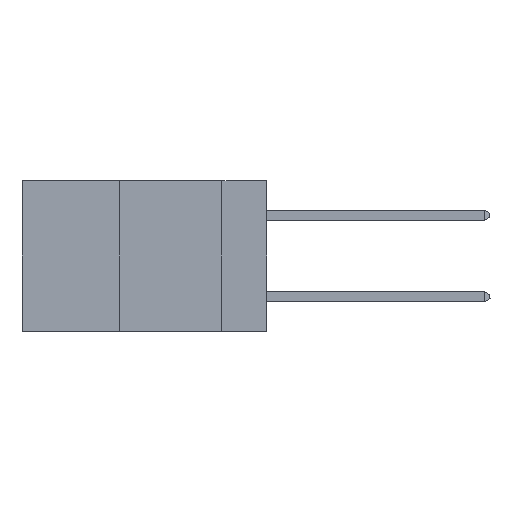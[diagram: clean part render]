
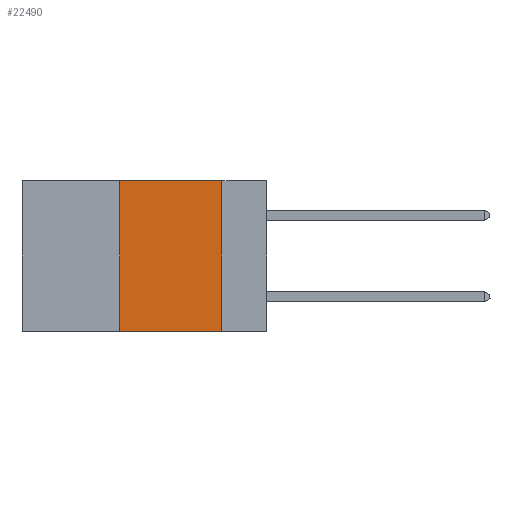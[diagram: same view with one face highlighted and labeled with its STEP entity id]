
A CAD part, left-side view. The second image highlights one B-rep face of the part: STEP entity #22490.
In plain terms, the highlighted planar face has unit normal (-1, 0, 0).
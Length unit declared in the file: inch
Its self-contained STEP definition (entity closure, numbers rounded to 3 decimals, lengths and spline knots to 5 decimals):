
#367 = VECTOR ( 'NONE', #22513, 39.37008 ) ;
#1401 = CARTESIAN_POINT ( 'NONE',  ( 0., 0.6, -0.37 ) ) ;
#1449 = CARTESIAN_POINT ( 'NONE',  ( 0., 0.11, 0. ) ) ;
#2160 = DIRECTION ( 'NONE',  ( 0., 0., -1. ) ) ;
#3634 = EDGE_CURVE ( 'NONE', #8290, #9306, #16051, .T. ) ;
#5881 = CARTESIAN_POINT ( 'NONE',  ( 0., 0.6, 0. ) ) ;
#7164 = EDGE_CURVE ( 'NONE', #9306, #13110, #24698, .T. ) ;
#7199 = FACE_OUTER_BOUND ( 'NONE', #22809, .T. ) ;
#7933 = DIRECTION ( 'NONE',  ( 1., 0., 0. ) ) ;
#8290 = VERTEX_POINT ( 'NONE', #11696 ) ;
#8476 = VECTOR ( 'NONE', #19211, 39.37008 ) ;
#8599 = CARTESIAN_POINT ( 'NONE',  ( 0., 0.11, -0.37 ) ) ;
#9306 = VERTEX_POINT ( 'NONE', #1449 ) ;
#9375 = CARTESIAN_POINT ( 'NONE',  ( 0., 0.36, -0.37 ) ) ;
#11696 = CARTESIAN_POINT ( 'NONE',  ( 0., 0.36, 0. ) ) ;
#12373 = CARTESIAN_POINT ( 'NONE',  ( 0., 0.11, 0. ) ) ;
#12525 = VECTOR ( 'NONE', #17699, 39.37008 ) ;
#13110 = VERTEX_POINT ( 'NONE', #8599 ) ;
#14006 = EDGE_CURVE ( 'NONE', #24593, #8290, #17898, .T. ) ;
#14942 = VECTOR ( 'NONE', #2160, 39.37008 ) ;
#15352 = EDGE_CURVE ( 'NONE', #24593, #13110, #22393, .T. ) ;
#16051 = LINE ( 'NONE', #23934, #367 ) ;
#17699 = DIRECTION ( 'NONE',  ( 0., -1., 0. ) ) ;
#17898 = LINE ( 'NONE', #21150, #8476 ) ;
#17974 = PLANE ( 'NONE',  #25575 ) ;
#19211 = DIRECTION ( 'NONE',  ( 0., 0., 1. ) ) ;
#20275 = ORIENTED_EDGE ( 'NONE', *, *, #3634, .F. ) ;
#20504 = ORIENTED_EDGE ( 'NONE', *, *, #7164, .F. ) ;
#21150 = CARTESIAN_POINT ( 'NONE',  ( 0., 0.36, 0. ) ) ;
#21880 = DIRECTION ( 'NONE',  ( 0., 0., -1. ) ) ;
#22393 = LINE ( 'NONE', #1401, #12525 ) ;
#22490 = ADVANCED_FACE ( 'NONE', ( #7199 ), #17974, .F. ) ;
#22513 = DIRECTION ( 'NONE',  ( 0., -1., 0. ) ) ;
#22708 = ORIENTED_EDGE ( 'NONE', *, *, #15352, .T. ) ;
#22809 = EDGE_LOOP ( 'NONE', ( #20504, #20275, #22950, #22708 ) ) ;
#22950 = ORIENTED_EDGE ( 'NONE', *, *, #14006, .F. ) ;
#23934 = CARTESIAN_POINT ( 'NONE',  ( 0., 0.6, 0. ) ) ;
#24593 = VERTEX_POINT ( 'NONE', #9375 ) ;
#24698 = LINE ( 'NONE', #12373, #14942 ) ;
#25575 = AXIS2_PLACEMENT_3D ( 'NONE', #5881, #7933, #21880 ) ;
